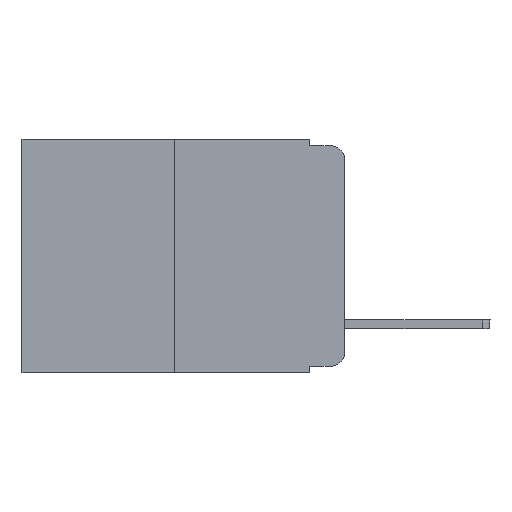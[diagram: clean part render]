
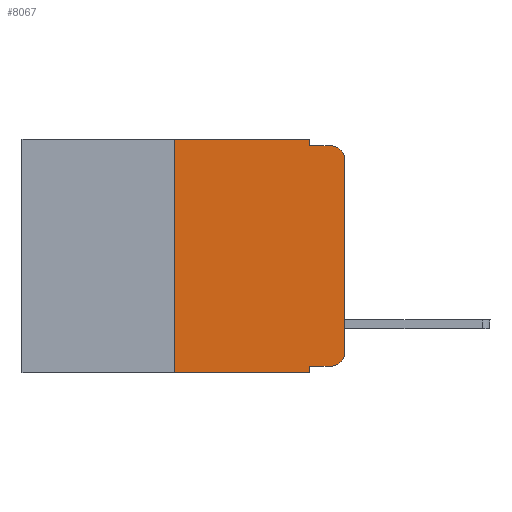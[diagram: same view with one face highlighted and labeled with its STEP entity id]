
A CAD part, left-side view. The second image highlights one B-rep face of the part: STEP entity #8067.
In plain terms, the highlighted planar face has unit normal (-1, 0, 0).
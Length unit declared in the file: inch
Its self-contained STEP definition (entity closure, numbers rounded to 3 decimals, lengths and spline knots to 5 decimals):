
#194 = CARTESIAN_POINT ( 'NONE',  ( 0., 0.051, 0. ) ) ;
#546 = EDGE_CURVE ( 'NONE', #6956, #6722, #15398, .T. ) ;
#694 = FACE_OUTER_BOUND ( 'NONE', #8354, .T. ) ;
#926 = DIRECTION ( 'NONE',  ( -1., 0., 0. ) ) ;
#1091 = VERTEX_POINT ( 'NONE', #12271 ) ;
#1291 = VERTEX_POINT ( 'NONE', #14092 ) ;
#1330 = LINE ( 'NONE', #4228, #15917 ) ;
#1524 = EDGE_CURVE ( 'NONE', #6722, #3762, #4132, .T. ) ;
#1800 = CARTESIAN_POINT ( 'NONE',  ( 0., 0., 0. ) ) ;
#1877 = ORIENTED_EDGE ( 'NONE', *, *, #6245, .T. ) ;
#2078 = DIRECTION ( 'NONE',  ( 0., 0., 1. ) ) ;
#2107 = CIRCLE ( 'NONE', #16120, 0.02 ) ;
#2166 = EDGE_CURVE ( 'NONE', #8745, #15289, #11095, .T. ) ;
#2349 = DIRECTION ( 'NONE',  ( 0., 0., -1. ) ) ;
#2604 = CARTESIAN_POINT ( 'NONE',  ( 0., 0., -0.03 ) ) ;
#2629 = LINE ( 'NONE', #6585, #6187 ) ;
#3109 = ORIENTED_EDGE ( 'NONE', *, *, #11120, .F. ) ;
#3250 = CARTESIAN_POINT ( 'NONE',  ( 0., 0.473, 0. ) ) ;
#3422 = DIRECTION ( 'NONE',  ( 0., 0., -1. ) ) ;
#3451 = CARTESIAN_POINT ( 'NONE',  ( 0., 0.02, -0.333 ) ) ;
#3485 = CARTESIAN_POINT ( 'NONE',  ( 0., 0.051, 0. ) ) ;
#3762 = VERTEX_POINT ( 'NONE', #194 ) ;
#3893 = VECTOR ( 'NONE', #7518, 39.37008 ) ;
#3909 = ORIENTED_EDGE ( 'NONE', *, *, #13280, .T. ) ;
#4067 = EDGE_CURVE ( 'NONE', #13135, #1291, #2629, .T. ) ;
#4132 = LINE ( 'NONE', #9467, #4534 ) ;
#4228 = CARTESIAN_POINT ( 'NONE',  ( 0., 0.051, -0.333 ) ) ;
#4404 = DIRECTION ( 'NONE',  ( -1., 0., 0. ) ) ;
#4485 = PLANE ( 'NONE',  #14677 ) ;
#4534 = VECTOR ( 'NONE', #14893, 39.37008 ) ;
#4957 = CARTESIAN_POINT ( 'NONE',  ( 0., 0.25, 0. ) ) ;
#5080 = CARTESIAN_POINT ( 'NONE',  ( 0., 0.473, -0.343 ) ) ;
#5194 = VERTEX_POINT ( 'NONE', #3451 ) ;
#6187 = VECTOR ( 'NONE', #14723, 39.37008 ) ;
#6245 = EDGE_CURVE ( 'NONE', #15289, #7944, #6532, .T. ) ;
#6532 = CIRCLE ( 'NONE', #13765, 0.02 ) ;
#6585 = CARTESIAN_POINT ( 'NONE',  ( 0., 0.051, 0. ) ) ;
#6722 = VERTEX_POINT ( 'NONE', #4957 ) ;
#6741 = ORIENTED_EDGE ( 'NONE', *, *, #16708, .F. ) ;
#6956 = VERTEX_POINT ( 'NONE', #13507 ) ;
#7442 = ORIENTED_EDGE ( 'NONE', *, *, #13887, .T. ) ;
#7518 = DIRECTION ( 'NONE',  ( 0., -1., 0. ) ) ;
#7944 = VERTEX_POINT ( 'NONE', #8248 ) ;
#8067 = ADVANCED_FACE ( 'NONE', ( #694 ), #4485, .F. ) ;
#8248 = CARTESIAN_POINT ( 'NONE',  ( 0., 0.02, -0.01 ) ) ;
#8354 = EDGE_LOOP ( 'NONE', ( #8568, #1877, #6741, #3109, #13393, #17199, #7442, #13927, #3909, #15704 ) ) ;
#8568 = ORIENTED_EDGE ( 'NONE', *, *, #2166, .T. ) ;
#8731 = DIRECTION ( 'NONE',  ( 0., 0., -1. ) ) ;
#8745 = VERTEX_POINT ( 'NONE', #10473 ) ;
#9219 = CARTESIAN_POINT ( 'NONE',  ( 0., 0.051, -0.333 ) ) ;
#9237 = LINE ( 'NONE', #14574, #15610 ) ;
#9467 = CARTESIAN_POINT ( 'NONE',  ( 0., 0.473, 0. ) ) ;
#10409 = LINE ( 'NONE', #5080, #3893 ) ;
#10473 = CARTESIAN_POINT ( 'NONE',  ( 0., 0., -0.313 ) ) ;
#11043 = DIRECTION ( 'NONE',  ( 0., -1., 0. ) ) ;
#11095 = LINE ( 'NONE', #1800, #12837 ) ;
#11120 = EDGE_CURVE ( 'NONE', #3762, #1091, #14434, .T. ) ;
#12271 = CARTESIAN_POINT ( 'NONE',  ( 0., 0.051, -0.01 ) ) ;
#12478 = DIRECTION ( 'NONE',  ( 0., 0., 1. ) ) ;
#12837 = VECTOR ( 'NONE', #12478, 39.37008 ) ;
#12922 = CARTESIAN_POINT ( 'NONE',  ( 0., 0.02, -0.03 ) ) ;
#13135 = VERTEX_POINT ( 'NONE', #9219 ) ;
#13280 = EDGE_CURVE ( 'NONE', #13135, #5194, #1330, .T. ) ;
#13342 = DIRECTION ( 'NONE',  ( 0., -1., 0. ) ) ;
#13393 = ORIENTED_EDGE ( 'NONE', *, *, #1524, .F. ) ;
#13507 = CARTESIAN_POINT ( 'NONE',  ( 0., 0.25, -0.343 ) ) ;
#13759 = VECTOR ( 'NONE', #2078, 39.37008 ) ;
#13765 = AXIS2_PLACEMENT_3D ( 'NONE', #12922, #926, #8731 ) ;
#13887 = EDGE_CURVE ( 'NONE', #6956, #1291, #10409, .T. ) ;
#13927 = ORIENTED_EDGE ( 'NONE', *, *, #4067, .F. ) ;
#14069 = CARTESIAN_POINT ( 'NONE',  ( 0., 0.25, 0. ) ) ;
#14092 = CARTESIAN_POINT ( 'NONE',  ( 0., 0.051, -0.343 ) ) ;
#14410 = EDGE_CURVE ( 'NONE', #5194, #8745, #2107, .T. ) ;
#14434 = LINE ( 'NONE', #3485, #16692 ) ;
#14574 = CARTESIAN_POINT ( 'NONE',  ( 0., 0.051, -0.01 ) ) ;
#14677 = AXIS2_PLACEMENT_3D ( 'NONE', #3250, #15425, #3422 ) ;
#14723 = DIRECTION ( 'NONE',  ( 0., 0., -1. ) ) ;
#14893 = DIRECTION ( 'NONE',  ( 0., -1., 0. ) ) ;
#14996 = CARTESIAN_POINT ( 'NONE',  ( 0., 0.02, -0.313 ) ) ;
#15289 = VERTEX_POINT ( 'NONE', #2604 ) ;
#15398 = LINE ( 'NONE', #14069, #13759 ) ;
#15425 = DIRECTION ( 'NONE',  ( 1., 0., 0. ) ) ;
#15610 = VECTOR ( 'NONE', #13342, 39.37008 ) ;
#15704 = ORIENTED_EDGE ( 'NONE', *, *, #14410, .T. ) ;
#15917 = VECTOR ( 'NONE', #11043, 39.37008 ) ;
#16120 = AXIS2_PLACEMENT_3D ( 'NONE', #14996, #4404, #16414 ) ;
#16414 = DIRECTION ( 'NONE',  ( 0., 0., -1. ) ) ;
#16692 = VECTOR ( 'NONE', #2349, 39.37008 ) ;
#16708 = EDGE_CURVE ( 'NONE', #1091, #7944, #9237, .T. ) ;
#17199 = ORIENTED_EDGE ( 'NONE', *, *, #546, .F. ) ;
